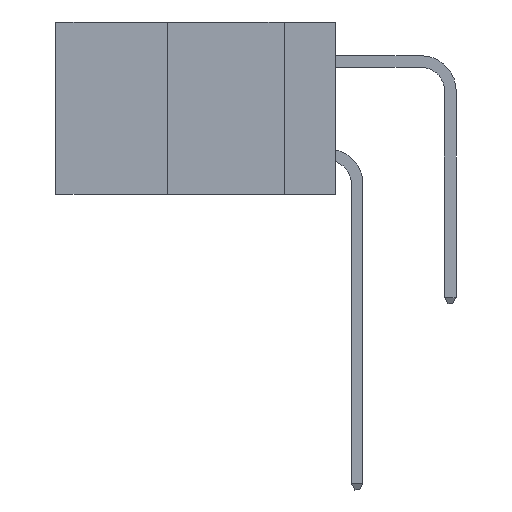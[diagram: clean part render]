
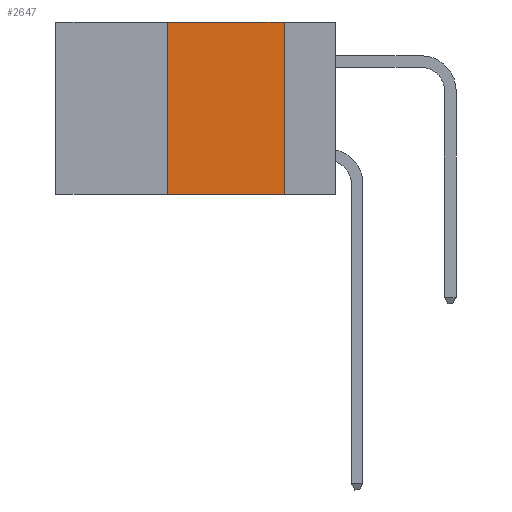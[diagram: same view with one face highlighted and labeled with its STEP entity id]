
A CAD part, left-side view. The second image highlights one B-rep face of the part: STEP entity #2647.
In plain terms, the highlighted planar face has unit normal (-1, 0, 0).
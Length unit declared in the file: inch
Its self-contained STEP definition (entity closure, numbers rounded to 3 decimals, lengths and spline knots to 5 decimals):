
#169 = CARTESIAN_POINT ( 'NONE',  ( 0., 0.6, -0.37 ) ) ;
#383 = DIRECTION ( 'NONE',  ( 1., 0., 0. ) ) ;
#638 = CARTESIAN_POINT ( 'NONE',  ( 0., 0.11, -0.37 ) ) ;
#685 = VERTEX_POINT ( 'NONE', #638 ) ;
#752 = EDGE_LOOP ( 'NONE', ( #8842, #8564, #4299, #3577 ) ) ;
#776 = LINE ( 'NONE', #9974, #2706 ) ;
#1204 = CARTESIAN_POINT ( 'NONE',  ( 0., 0.6, 0. ) ) ;
#2134 = LINE ( 'NONE', #8929, #3071 ) ;
#2209 = DIRECTION ( 'NONE',  ( 0., 0., -1. ) ) ;
#2287 = EDGE_CURVE ( 'NONE', #8160, #10226, #776, .T. ) ;
#2333 = CARTESIAN_POINT ( 'NONE',  ( 0., 0.36, -0.37 ) ) ;
#2647 = ADVANCED_FACE ( 'NONE', ( #6528 ), #2652, .F. ) ;
#2652 = PLANE ( 'NONE',  #5724 ) ;
#2693 = DIRECTION ( 'NONE',  ( 0., -1., 0. ) ) ;
#2706 = VECTOR ( 'NONE', #4593, 39.37008 ) ;
#2772 = LINE ( 'NONE', #169, #6061 ) ;
#2929 = CARTESIAN_POINT ( 'NONE',  ( 0., 0.36, 0. ) ) ;
#3071 = VECTOR ( 'NONE', #10624, 39.37008 ) ;
#3573 = EDGE_CURVE ( 'NONE', #3972, #8160, #7215, .T. ) ;
#3577 = ORIENTED_EDGE ( 'NONE', *, *, #10077, .T. ) ;
#3711 = CARTESIAN_POINT ( 'NONE',  ( 0., 0.11, 0. ) ) ;
#3780 = EDGE_CURVE ( 'NONE', #10226, #685, #2134, .T. ) ;
#3972 = VERTEX_POINT ( 'NONE', #2333 ) ;
#4062 = CARTESIAN_POINT ( 'NONE',  ( 0., 0.36, 0. ) ) ;
#4299 = ORIENTED_EDGE ( 'NONE', *, *, #3573, .F. ) ;
#4593 = DIRECTION ( 'NONE',  ( 0., -1., 0. ) ) ;
#5724 = AXIS2_PLACEMENT_3D ( 'NONE', #1204, #383, #2209 ) ;
#6061 = VECTOR ( 'NONE', #2693, 39.37008 ) ;
#6528 = FACE_OUTER_BOUND ( 'NONE', #752, .T. ) ;
#7215 = LINE ( 'NONE', #4062, #11186 ) ;
#8160 = VERTEX_POINT ( 'NONE', #2929 ) ;
#8564 = ORIENTED_EDGE ( 'NONE', *, *, #2287, .F. ) ;
#8842 = ORIENTED_EDGE ( 'NONE', *, *, #3780, .F. ) ;
#8929 = CARTESIAN_POINT ( 'NONE',  ( 0., 0.11, 0. ) ) ;
#9974 = CARTESIAN_POINT ( 'NONE',  ( 0., 0.6, 0. ) ) ;
#10077 = EDGE_CURVE ( 'NONE', #3972, #685, #2772, .T. ) ;
#10226 = VERTEX_POINT ( 'NONE', #3711 ) ;
#10624 = DIRECTION ( 'NONE',  ( 0., 0., -1. ) ) ;
#11066 = DIRECTION ( 'NONE',  ( 0., 0., 1. ) ) ;
#11186 = VECTOR ( 'NONE', #11066, 39.37008 ) ;
